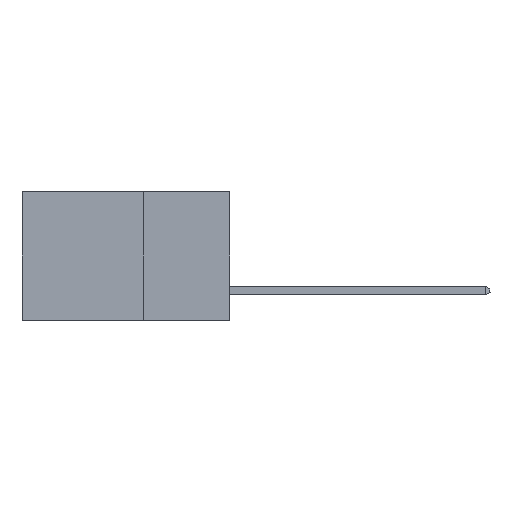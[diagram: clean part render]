
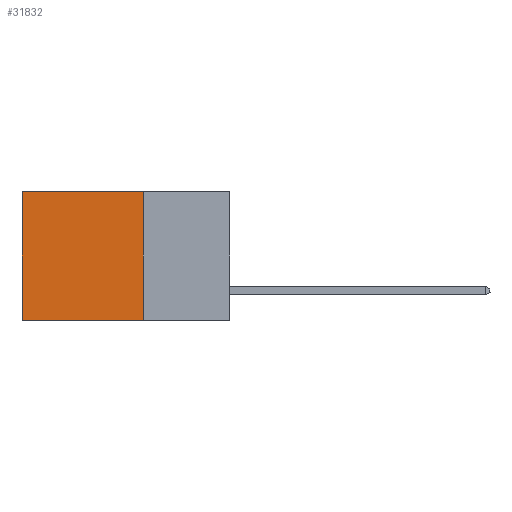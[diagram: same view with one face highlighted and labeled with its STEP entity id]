
A CAD part, left-side view. The second image highlights one B-rep face of the part: STEP entity #31832.
In plain terms, the highlighted planar face has unit normal (-1, 0, 0).
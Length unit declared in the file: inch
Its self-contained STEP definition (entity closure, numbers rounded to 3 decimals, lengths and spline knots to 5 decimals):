
#355 = FACE_OUTER_BOUND ( 'NONE', #19051, .T. ) ;
#923 = DIRECTION ( 'NONE',  ( 0., 0., -1. ) ) ;
#2683 = LINE ( 'NONE', #6681, #31434 ) ;
#4888 = VERTEX_POINT ( 'NONE', #31295 ) ;
#5623 = VECTOR ( 'NONE', #26431, 39.37008 ) ;
#6681 = CARTESIAN_POINT ( 'NONE',  ( 0.298, 0.25, -0.37 ) ) ;
#7268 = CARTESIAN_POINT ( 'NONE',  ( 0.298, 0.25, 0. ) ) ;
#8027 = EDGE_CURVE ( 'NONE', #4888, #23363, #14105, .T. ) ;
#8202 = ORIENTED_EDGE ( 'NONE', *, *, #8027, .T. ) ;
#8527 = DIRECTION ( 'NONE',  ( 0., 0., -1. ) ) ;
#9000 = ORIENTED_EDGE ( 'NONE', *, *, #24379, .F. ) ;
#9564 = VECTOR ( 'NONE', #21956, 39.37008 ) ;
#9577 = VERTEX_POINT ( 'NONE', #21012 ) ;
#11075 = DIRECTION ( 'NONE',  ( 1., 0., 0. ) ) ;
#14105 = LINE ( 'NONE', #19890, #9564 ) ;
#15635 = ORIENTED_EDGE ( 'NONE', *, *, #24072, .T. ) ;
#16326 = VECTOR ( 'NONE', #923, 39.37008 ) ;
#16638 = ORIENTED_EDGE ( 'NONE', *, *, #29118, .F. ) ;
#17161 = CARTESIAN_POINT ( 'NONE',  ( 0.298, 0.6, 0. ) ) ;
#18156 = CARTESIAN_POINT ( 'NONE',  ( 0.298, 0.6, 0. ) ) ;
#18236 = LINE ( 'NONE', #7268, #5623 ) ;
#19051 = EDGE_LOOP ( 'NONE', ( #15635, #16638, #9000, #8202 ) ) ;
#19890 = CARTESIAN_POINT ( 'NONE',  ( 0.298, 0.25, 0. ) ) ;
#21012 = CARTESIAN_POINT ( 'NONE',  ( 0.298, 0.6, -0.37 ) ) ;
#21956 = DIRECTION ( 'NONE',  ( 0., 1., 0. ) ) ;
#21981 = VERTEX_POINT ( 'NONE', #26277 ) ;
#22878 = LINE ( 'NONE', #18156, #16326 ) ;
#23177 = CARTESIAN_POINT ( 'NONE',  ( 0.298, 0.25, 0. ) ) ;
#23363 = VERTEX_POINT ( 'NONE', #17161 ) ;
#24072 = EDGE_CURVE ( 'NONE', #23363, #9577, #22878, .T. ) ;
#24151 = DIRECTION ( 'NONE',  ( 0., 1., 0. ) ) ;
#24379 = EDGE_CURVE ( 'NONE', #4888, #21981, #18236, .T. ) ;
#25200 = AXIS2_PLACEMENT_3D ( 'NONE', #23177, #11075, #8527 ) ;
#26277 = CARTESIAN_POINT ( 'NONE',  ( 0.298, 0.25, -0.37 ) ) ;
#26431 = DIRECTION ( 'NONE',  ( 0., 0., -1. ) ) ;
#28357 = PLANE ( 'NONE',  #25200 ) ;
#29118 = EDGE_CURVE ( 'NONE', #21981, #9577, #2683, .T. ) ;
#31295 = CARTESIAN_POINT ( 'NONE',  ( 0.298, 0.25, 0. ) ) ;
#31434 = VECTOR ( 'NONE', #24151, 39.37008 ) ;
#31832 = ADVANCED_FACE ( 'NONE', ( #355 ), #28357, .F. ) ;
